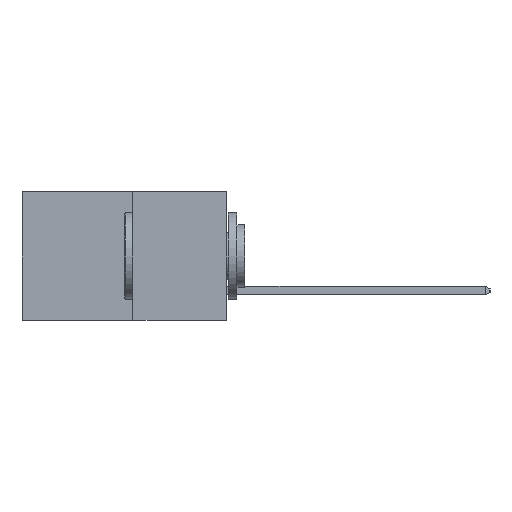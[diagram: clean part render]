
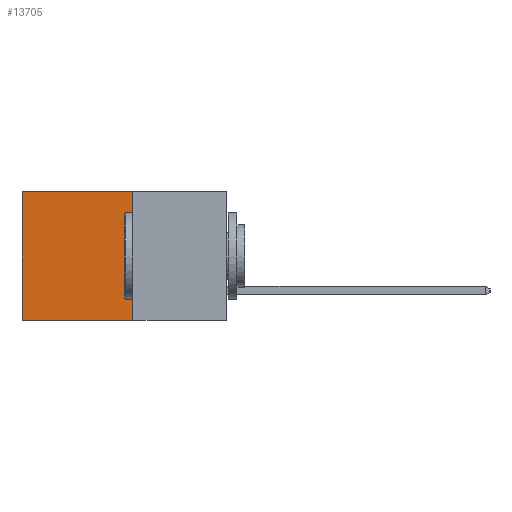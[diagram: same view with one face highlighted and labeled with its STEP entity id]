
A CAD part, left-side view. The second image highlights one B-rep face of the part: STEP entity #13705.
In plain terms, the highlighted planar face has unit normal (-1, 0, 0).
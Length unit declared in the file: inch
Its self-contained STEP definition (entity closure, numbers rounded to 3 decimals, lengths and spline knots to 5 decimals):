
#400 = LINE ( 'NONE', #4747, #12869 ) ;
#1057 = VECTOR ( 'NONE', #7207, 39.37008 ) ;
#1384 = CARTESIAN_POINT ( 'NONE',  ( 0.277, 0.59, -0.37 ) ) ;
#1972 = LINE ( 'NONE', #13872, #19256 ) ;
#3591 = CARTESIAN_POINT ( 'NONE',  ( 0.277, 0.27, 0. ) ) ;
#3797 = EDGE_CURVE ( 'NONE', #16344, #20776, #6196, .T. ) ;
#4213 = CARTESIAN_POINT ( 'NONE',  ( 0.277, 0.27, -0.37 ) ) ;
#4585 = CARTESIAN_POINT ( 'NONE',  ( 0.277, 0.27, 0. ) ) ;
#4747 = CARTESIAN_POINT ( 'NONE',  ( 0.277, 0.27, -0.37 ) ) ;
#5345 = ORIENTED_EDGE ( 'NONE', *, *, #3797, .T. ) ;
#5579 = DIRECTION ( 'NONE',  ( 0., 1., 0. ) ) ;
#6036 = PLANE ( 'NONE',  #10387 ) ;
#6196 = LINE ( 'NONE', #1384, #1057 ) ;
#6937 = EDGE_CURVE ( 'NONE', #12158, #17549, #400, .T. ) ;
#7207 = DIRECTION ( 'NONE',  ( 0., 0., -1. ) ) ;
#7725 = DIRECTION ( 'NONE',  ( 1., 0., 0. ) ) ;
#8110 = VECTOR ( 'NONE', #17909, 39.37008 ) ;
#8665 = CARTESIAN_POINT ( 'NONE',  ( 0.277, 0.27, -0.37 ) ) ;
#9547 = ORIENTED_EDGE ( 'NONE', *, *, #6937, .F. ) ;
#9864 = DIRECTION ( 'NONE',  ( 0., 0., -1. ) ) ;
#10387 = AXIS2_PLACEMENT_3D ( 'NONE', #4213, #7725, #19295 ) ;
#12158 = VERTEX_POINT ( 'NONE', #3591 ) ;
#12869 = VECTOR ( 'NONE', #9864, 39.37008 ) ;
#12910 = ORIENTED_EDGE ( 'NONE', *, *, #13581, .F. ) ;
#13025 = CARTESIAN_POINT ( 'NONE',  ( 0.277, 0.59, -0.37 ) ) ;
#13581 = EDGE_CURVE ( 'NONE', #17549, #20776, #1972, .T. ) ;
#13705 = ADVANCED_FACE ( 'NONE', ( #21063 ), #6036, .F. ) ;
#13872 = CARTESIAN_POINT ( 'NONE',  ( 0.277, 0.27, -0.37 ) ) ;
#14411 = EDGE_CURVE ( 'NONE', #12158, #16344, #21281, .T. ) ;
#16239 = ORIENTED_EDGE ( 'NONE', *, *, #14411, .T. ) ;
#16344 = VERTEX_POINT ( 'NONE', #20033 ) ;
#17549 = VERTEX_POINT ( 'NONE', #8665 ) ;
#17909 = DIRECTION ( 'NONE',  ( 0., 1., 0. ) ) ;
#18899 = EDGE_LOOP ( 'NONE', ( #5345, #12910, #9547, #16239 ) ) ;
#19256 = VECTOR ( 'NONE', #5579, 39.37008 ) ;
#19295 = DIRECTION ( 'NONE',  ( 0., 0., -1. ) ) ;
#20033 = CARTESIAN_POINT ( 'NONE',  ( 0.277, 0.59, 0. ) ) ;
#20776 = VERTEX_POINT ( 'NONE', #13025 ) ;
#21063 = FACE_OUTER_BOUND ( 'NONE', #18899, .T. ) ;
#21281 = LINE ( 'NONE', #4585, #8110 ) ;
